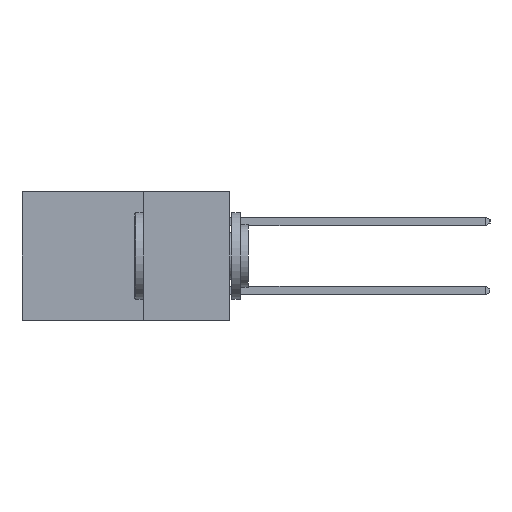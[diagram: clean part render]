
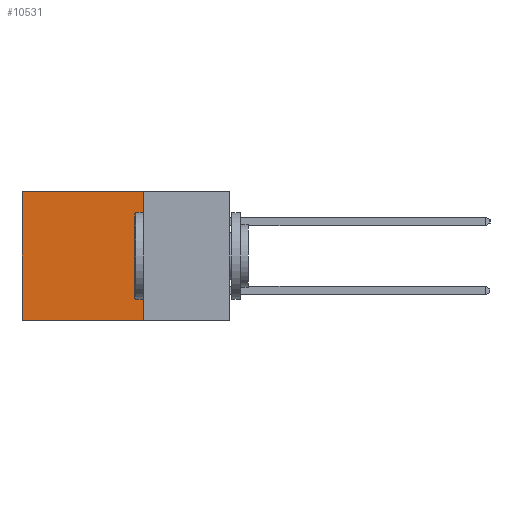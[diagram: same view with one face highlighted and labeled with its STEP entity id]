
A CAD part, left-side view. The second image highlights one B-rep face of the part: STEP entity #10531.
In plain terms, the highlighted planar face has unit normal (-1, 0, 0).
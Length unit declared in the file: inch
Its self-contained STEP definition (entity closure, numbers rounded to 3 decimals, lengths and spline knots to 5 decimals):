
#370 = FACE_OUTER_BOUND ( 'NONE', #2553, .T. ) ;
#1936 = ORIENTED_EDGE ( 'NONE', *, *, #10641, .F. ) ;
#2553 = EDGE_LOOP ( 'NONE', ( #3319, #1936, #15152, #20403 ) ) ;
#2968 = AXIS2_PLACEMENT_3D ( 'NONE', #21288, #5135, #17758 ) ;
#3124 = CARTESIAN_POINT ( 'NONE',  ( 0.298, 0.25, -0.37 ) ) ;
#3229 = PLANE ( 'NONE',  #2968 ) ;
#3284 = LINE ( 'NONE', #4405, #21945 ) ;
#3319 = ORIENTED_EDGE ( 'NONE', *, *, #4376, .T. ) ;
#3554 = DIRECTION ( 'NONE',  ( 0., 1., 0. ) ) ;
#4376 = EDGE_CURVE ( 'NONE', #8936, #6678, #3284, .T. ) ;
#4405 = CARTESIAN_POINT ( 'NONE',  ( 0.298, 0.6, 0. ) ) ;
#5094 = VERTEX_POINT ( 'NONE', #3124 ) ;
#5135 = DIRECTION ( 'NONE',  ( 1., 0., 0. ) ) ;
#6678 = VERTEX_POINT ( 'NONE', #15885 ) ;
#7220 = VECTOR ( 'NONE', #23236, 39.37008 ) ;
#7310 = VECTOR ( 'NONE', #3554, 39.37008 ) ;
#7502 = EDGE_CURVE ( 'NONE', #19584, #5094, #13143, .T. ) ;
#8936 = VERTEX_POINT ( 'NONE', #9861 ) ;
#9861 = CARTESIAN_POINT ( 'NONE',  ( 0.298, 0.6, 0. ) ) ;
#10531 = ADVANCED_FACE ( 'NONE', ( #370 ), #3229, .F. ) ;
#10641 = EDGE_CURVE ( 'NONE', #5094, #6678, #21090, .T. ) ;
#12016 = LINE ( 'NONE', #21507, #7220 ) ;
#13143 = LINE ( 'NONE', #14337, #17932 ) ;
#13774 = CARTESIAN_POINT ( 'NONE',  ( 0.298, 0.25, 0. ) ) ;
#14337 = CARTESIAN_POINT ( 'NONE',  ( 0.298, 0.25, 0. ) ) ;
#14983 = DIRECTION ( 'NONE',  ( 0., 0., -1. ) ) ;
#15152 = ORIENTED_EDGE ( 'NONE', *, *, #7502, .F. ) ;
#15885 = CARTESIAN_POINT ( 'NONE',  ( 0.298, 0.6, -0.37 ) ) ;
#17758 = DIRECTION ( 'NONE',  ( 0., 0., -1. ) ) ;
#17932 = VECTOR ( 'NONE', #14983, 39.37008 ) ;
#18072 = CARTESIAN_POINT ( 'NONE',  ( 0.298, 0.25, -0.37 ) ) ;
#19381 = DIRECTION ( 'NONE',  ( 0., 0., -1. ) ) ;
#19584 = VERTEX_POINT ( 'NONE', #13774 ) ;
#20403 = ORIENTED_EDGE ( 'NONE', *, *, #21488, .T. ) ;
#21090 = LINE ( 'NONE', #18072, #7310 ) ;
#21288 = CARTESIAN_POINT ( 'NONE',  ( 0.298, 0.25, 0. ) ) ;
#21488 = EDGE_CURVE ( 'NONE', #19584, #8936, #12016, .T. ) ;
#21507 = CARTESIAN_POINT ( 'NONE',  ( 0.298, 0.25, 0. ) ) ;
#21945 = VECTOR ( 'NONE', #19381, 39.37008 ) ;
#23236 = DIRECTION ( 'NONE',  ( 0., 1., 0. ) ) ;
